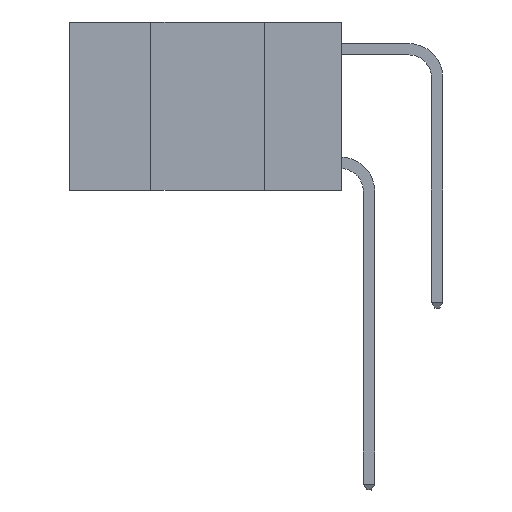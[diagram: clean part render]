
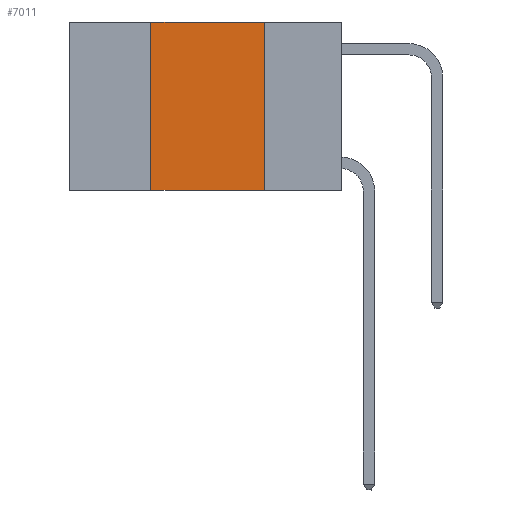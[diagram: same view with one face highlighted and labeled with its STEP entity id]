
A CAD part, left-side view. The second image highlights one B-rep face of the part: STEP entity #7011.
In plain terms, the highlighted planar face has unit normal (-1, 0, 0).
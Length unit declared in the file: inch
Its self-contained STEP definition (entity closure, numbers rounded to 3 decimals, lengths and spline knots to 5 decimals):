
#627 = VERTEX_POINT ( 'NONE', #9738 ) ;
#1421 = DIRECTION ( 'NONE',  ( 1., 0., 0. ) ) ;
#1516 = EDGE_CURVE ( 'NONE', #10675, #627, #3540, .T. ) ;
#1650 = ORIENTED_EDGE ( 'NONE', *, *, #1696, .T. ) ;
#1696 = EDGE_CURVE ( 'NONE', #8031, #3533, #2275, .T. ) ;
#2133 = DIRECTION ( 'NONE',  ( 0., 0., -1. ) ) ;
#2265 = ORIENTED_EDGE ( 'NONE', *, *, #1516, .F. ) ;
#2275 = LINE ( 'NONE', #11226, #9583 ) ;
#2850 = CARTESIAN_POINT ( 'NONE',  ( 0., 0.17, 0. ) ) ;
#3533 = VERTEX_POINT ( 'NONE', #3869 ) ;
#3540 = LINE ( 'NONE', #10758, #8732 ) ;
#3830 = CARTESIAN_POINT ( 'NONE',  ( 0., 0.42, -0.37 ) ) ;
#3869 = CARTESIAN_POINT ( 'NONE',  ( 0., 0.17, -0.37 ) ) ;
#3924 = CARTESIAN_POINT ( 'NONE',  ( 0., 0.42, 0. ) ) ;
#4607 = AXIS2_PLACEMENT_3D ( 'NONE', #5260, #1421, #2133 ) ;
#5248 = ORIENTED_EDGE ( 'NONE', *, *, #7183, .F. ) ;
#5260 = CARTESIAN_POINT ( 'NONE',  ( 0., 0.6, 0. ) ) ;
#5819 = DIRECTION ( 'NONE',  ( 0., 0., 1. ) ) ;
#6431 = VECTOR ( 'NONE', #10559, 39.37008 ) ;
#7011 = ADVANCED_FACE ( 'NONE', ( #10246 ), #9122, .F. ) ;
#7183 = EDGE_CURVE ( 'NONE', #8031, #10675, #10398, .T. ) ;
#7894 = DIRECTION ( 'NONE',  ( 0., -1., 0. ) ) ;
#8031 = VERTEX_POINT ( 'NONE', #3830 ) ;
#8036 = ORIENTED_EDGE ( 'NONE', *, *, #10301, .F. ) ;
#8381 = DIRECTION ( 'NONE',  ( 0., -1., 0. ) ) ;
#8732 = VECTOR ( 'NONE', #7894, 39.37008 ) ;
#9122 = PLANE ( 'NONE',  #4607 ) ;
#9226 = EDGE_LOOP ( 'NONE', ( #8036, #2265, #5248, #1650 ) ) ;
#9551 = CARTESIAN_POINT ( 'NONE',  ( 0., 0.42, 0. ) ) ;
#9583 = VECTOR ( 'NONE', #8381, 39.37008 ) ;
#9738 = CARTESIAN_POINT ( 'NONE',  ( 0., 0.17, 0. ) ) ;
#10115 = VECTOR ( 'NONE', #5819, 39.37008 ) ;
#10246 = FACE_OUTER_BOUND ( 'NONE', #9226, .T. ) ;
#10301 = EDGE_CURVE ( 'NONE', #627, #3533, #11499, .T. ) ;
#10398 = LINE ( 'NONE', #9551, #10115 ) ;
#10559 = DIRECTION ( 'NONE',  ( 0., 0., -1. ) ) ;
#10675 = VERTEX_POINT ( 'NONE', #3924 ) ;
#10758 = CARTESIAN_POINT ( 'NONE',  ( 0., 0.6, 0. ) ) ;
#11226 = CARTESIAN_POINT ( 'NONE',  ( 0., 0.6, -0.37 ) ) ;
#11499 = LINE ( 'NONE', #2850, #6431 ) ;
